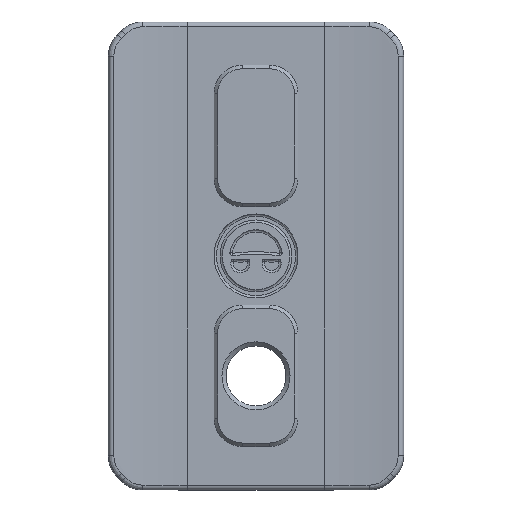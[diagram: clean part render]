
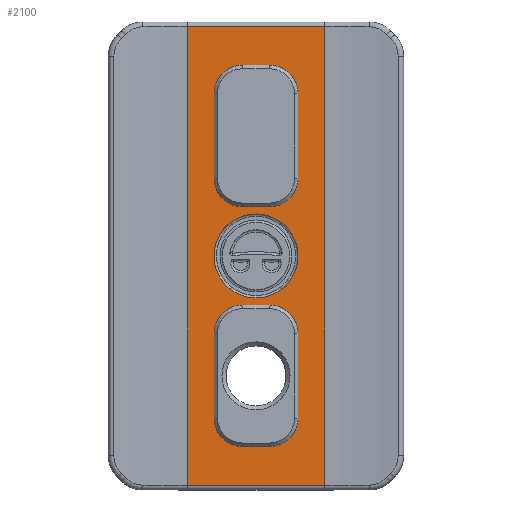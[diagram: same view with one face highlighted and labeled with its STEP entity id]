
A CAD part, top view. The second image highlights one B-rep face of the part: STEP entity #2100.
In plain terms, the highlighted planar face has unit normal (0, 0, 1).
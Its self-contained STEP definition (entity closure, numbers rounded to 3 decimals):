
#126=FACE_BOUND('',#397,.T.);
#127=FACE_BOUND('',#398,.T.);
#128=FACE_BOUND('',#399,.T.);
#199=PLANE('',#2283);
#251=FACE_OUTER_BOUND('',#396,.T.);
#396=EDGE_LOOP('',(#1549,#1550,#1551,#1552));
#397=EDGE_LOOP('',(#1553,#1554,#1555,#1556,#1557,#1558,#1559,#1560));
#398=EDGE_LOOP('',(#1561));
#399=EDGE_LOOP('',(#1562,#1563,#1564,#1565,#1566,#1567,#1568,#1569));
#525=CIRCLE('',#2244,2.38);
#526=CIRCLE('',#2247,2.38);
#535=CIRCLE('',#2266,2.38);
#536=CIRCLE('',#2269,2.38);
#538=CIRCLE('',#2274,2.38);
#539=CIRCLE('',#2277,2.38);
#540=CIRCLE('',#2279,2.38);
#541=CIRCLE('',#2282,2.38);
#542=CIRCLE('',#2284,3.5);
#677=LINE('',#3244,#797);
#681=LINE('',#3253,#801);
#702=LINE('',#3316,#822);
#705=LINE('',#3324,#825);
#709=LINE('',#3337,#829);
#712=LINE('',#3347,#832);
#714=LINE('',#3355,#834);
#715=LINE('',#3357,#835);
#716=LINE('',#3359,#836);
#717=LINE('',#3360,#837);
#718=LINE('',#3361,#838);
#719=LINE('',#3364,#839);
#797=VECTOR('',#2560,10.);
#801=VECTOR('',#2570,10.);
#822=VECTOR('',#2635,10.);
#825=VECTOR('',#2644,10.);
#829=VECTOR('',#2658,10.);
#832=VECTOR('',#2671,10.);
#834=VECTOR('',#2679,10.);
#835=VECTOR('',#2680,10.);
#836=VECTOR('',#2681,10.);
#837=VECTOR('',#2682,10.);
#838=VECTOR('',#2683,10.);
#839=VECTOR('',#2686,10.);
#916=VERTEX_POINT('',#3241);
#917=VERTEX_POINT('',#3243);
#918=VERTEX_POINT('',#3247);
#919=VERTEX_POINT('',#3251);
#920=VERTEX_POINT('',#3255);
#937=VERTEX_POINT('',#3308);
#938=VERTEX_POINT('',#3310);
#939=VERTEX_POINT('',#3314);
#940=VERTEX_POINT('',#3318);
#941=VERTEX_POINT('',#3322);
#943=VERTEX_POINT('',#3329);
#944=VERTEX_POINT('',#3331);
#945=VERTEX_POINT('',#3335);
#946=VERTEX_POINT('',#3341);
#947=VERTEX_POINT('',#3343);
#948=VERTEX_POINT('',#3349);
#949=VERTEX_POINT('',#3353);
#950=VERTEX_POINT('',#3354);
#951=VERTEX_POINT('',#3356);
#952=VERTEX_POINT('',#3358);
#953=VERTEX_POINT('',#3362);
#1114=EDGE_CURVE('',#916,#917,#677,.T.);
#1117=EDGE_CURVE('',#918,#916,#525,.F.);
#1119=EDGE_CURVE('',#919,#918,#681,.F.);
#1121=EDGE_CURVE('',#920,#919,#526,.F.);
#1147=EDGE_CURVE('',#937,#938,#535,.F.);
#1150=EDGE_CURVE('',#939,#937,#702,.T.);
#1152=EDGE_CURVE('',#940,#939,#536,.F.);
#1154=EDGE_CURVE('',#941,#940,#705,.T.);
#1157=EDGE_CURVE('',#943,#944,#538,.F.);
#1160=EDGE_CURVE('',#945,#943,#709,.F.);
#1161=EDGE_CURVE('',#917,#945,#539,.F.);
#1163=EDGE_CURVE('',#946,#947,#540,.F.);
#1165=EDGE_CURVE('',#938,#946,#712,.F.);
#1167=EDGE_CURVE('',#948,#941,#541,.F.);
#1168=EDGE_CURVE('',#949,#950,#714,.T.);
#1169=EDGE_CURVE('',#951,#950,#715,.T.);
#1170=EDGE_CURVE('',#952,#951,#716,.T.);
#1171=EDGE_CURVE('',#949,#952,#717,.T.);
#1172=EDGE_CURVE('',#947,#948,#718,.T.);
#1173=EDGE_CURVE('',#953,#953,#542,.T.);
#1174=EDGE_CURVE('',#944,#920,#719,.T.);
#1549=ORIENTED_EDGE('',*,*,#1168,.T.);
#1550=ORIENTED_EDGE('',*,*,#1169,.F.);
#1551=ORIENTED_EDGE('',*,*,#1170,.F.);
#1552=ORIENTED_EDGE('',*,*,#1171,.F.);
#1553=ORIENTED_EDGE('',*,*,#1165,.F.);
#1554=ORIENTED_EDGE('',*,*,#1147,.F.);
#1555=ORIENTED_EDGE('',*,*,#1150,.F.);
#1556=ORIENTED_EDGE('',*,*,#1152,.F.);
#1557=ORIENTED_EDGE('',*,*,#1154,.F.);
#1558=ORIENTED_EDGE('',*,*,#1167,.F.);
#1559=ORIENTED_EDGE('',*,*,#1172,.F.);
#1560=ORIENTED_EDGE('',*,*,#1163,.F.);
#1561=ORIENTED_EDGE('',*,*,#1173,.T.);
#1562=ORIENTED_EDGE('',*,*,#1160,.F.);
#1563=ORIENTED_EDGE('',*,*,#1161,.F.);
#1564=ORIENTED_EDGE('',*,*,#1114,.F.);
#1565=ORIENTED_EDGE('',*,*,#1117,.F.);
#1566=ORIENTED_EDGE('',*,*,#1119,.F.);
#1567=ORIENTED_EDGE('',*,*,#1121,.F.);
#1568=ORIENTED_EDGE('',*,*,#1174,.F.);
#1569=ORIENTED_EDGE('',*,*,#1157,.F.);
#2100=ADVANCED_FACE('',(#251,#126,#127,#128),#199,.T.);
#2244=AXIS2_PLACEMENT_3D('',#3249,#2565,#2566);
#2247=AXIS2_PLACEMENT_3D('',#3257,#2574,#2575);
#2266=AXIS2_PLACEMENT_3D('',#3311,#2629,#2630);
#2269=AXIS2_PLACEMENT_3D('',#3320,#2639,#2640);
#2274=AXIS2_PLACEMENT_3D('',#3332,#2652,#2653);
#2277=AXIS2_PLACEMENT_3D('',#3339,#2661,#2662);
#2279=AXIS2_PLACEMENT_3D('',#3344,#2666,#2667);
#2282=AXIS2_PLACEMENT_3D('',#3351,#2675,#2676);
#2283=AXIS2_PLACEMENT_3D('',#3352,#2677,#2678);
#2284=AXIS2_PLACEMENT_3D('',#3363,#2684,#2685);
#2560=DIRECTION('',(0.,-1.,0.));
#2565=DIRECTION('center_axis',(0.,0.,-1.));
#2566=DIRECTION('ref_axis',(-0.707,0.707,0.));
#2570=DIRECTION('',(1.,0.,0.));
#2574=DIRECTION('center_axis',(0.,0.,-1.));
#2575=DIRECTION('ref_axis',(0.707,0.707,0.));
#2629=DIRECTION('center_axis',(0.,0.,-1.));
#2630=DIRECTION('ref_axis',(-0.707,-0.707,0.));
#2635=DIRECTION('',(0.,-1.,0.));
#2639=DIRECTION('center_axis',(0.,0.,-1.));
#2640=DIRECTION('ref_axis',(-0.707,0.707,0.));
#2644=DIRECTION('',(-1.,0.,0.));
#2652=DIRECTION('center_axis',(0.,0.,-1.));
#2653=DIRECTION('ref_axis',(0.707,-0.707,0.));
#2658=DIRECTION('',(-1.,0.,0.));
#2661=DIRECTION('center_axis',(0.,0.,-1.));
#2662=DIRECTION('ref_axis',(-0.707,-0.707,0.));
#2666=DIRECTION('center_axis',(0.,0.,-1.));
#2667=DIRECTION('ref_axis',(0.707,-0.707,0.));
#2671=DIRECTION('',(-1.,0.,0.));
#2675=DIRECTION('center_axis',(0.,0.,-1.));
#2676=DIRECTION('ref_axis',(0.707,0.707,0.));
#2677=DIRECTION('center_axis',(0.,0.,1.));
#2678=DIRECTION('ref_axis',(1.,0.,0.));
#2679=DIRECTION('',(0.,-1.,0.));
#2680=DIRECTION('',(-1.,0.,0.));
#2681=DIRECTION('',(0.,-1.,0.));
#2682=DIRECTION('',(1.,0.,0.));
#2683=DIRECTION('',(0.,1.,0.));
#2684=DIRECTION('center_axis',(0.,0.,-1.));
#2685=DIRECTION('ref_axis',(-1.,0.,0.));
#2686=DIRECTION('',(0.,1.,0.));
#3241=CARTESIAN_POINT('',(-3.5,37.52,-2.8));
#3243=CARTESIAN_POINT('',(-3.5,30.48,-2.8));
#3244=CARTESIAN_POINT('',(-3.5,7.19,-2.8));
#3247=CARTESIAN_POINT('',(-1.12,39.9,-2.8));
#3249=CARTESIAN_POINT('Origin',(-1.12,37.52,-2.8));
#3251=CARTESIAN_POINT('',(1.12,39.9,-2.8));
#3253=CARTESIAN_POINT('',(-30.56,39.9,-2.8));
#3255=CARTESIAN_POINT('',(3.5,37.52,-2.8));
#3257=CARTESIAN_POINT('Origin',(1.12,37.52,-2.8));
#3308=CARTESIAN_POINT('',(-3.5,10.48,-2.8));
#3310=CARTESIAN_POINT('',(-1.12,8.1,-2.8));
#3311=CARTESIAN_POINT('Origin',(-1.12,10.48,-2.8));
#3314=CARTESIAN_POINT('',(-3.5,17.52,-2.8));
#3316=CARTESIAN_POINT('',(-3.5,-2.81,-2.8));
#3318=CARTESIAN_POINT('',(-1.12,19.9,-2.8));
#3320=CARTESIAN_POINT('Origin',(-1.12,17.52,-2.8));
#3322=CARTESIAN_POINT('',(1.12,19.9,-2.8));
#3324=CARTESIAN_POINT('',(-29.44,19.9,-2.8));
#3329=CARTESIAN_POINT('',(1.12,28.1,-2.8));
#3331=CARTESIAN_POINT('',(3.5,30.48,-2.8));
#3332=CARTESIAN_POINT('Origin',(1.12,30.48,-2.8));
#3335=CARTESIAN_POINT('',(-1.12,28.1,-2.8));
#3337=CARTESIAN_POINT('',(-29.44,28.1,-2.8));
#3339=CARTESIAN_POINT('Origin',(-1.12,30.48,-2.8));
#3341=CARTESIAN_POINT('',(1.12,8.1,-2.8));
#3343=CARTESIAN_POINT('',(3.5,10.48,-2.8));
#3344=CARTESIAN_POINT('Origin',(1.12,10.48,-2.8));
#3347=CARTESIAN_POINT('',(-29.44,8.1,-2.8));
#3349=CARTESIAN_POINT('',(3.5,17.52,-2.8));
#3351=CARTESIAN_POINT('Origin',(1.12,17.52,-2.8));
#3352=CARTESIAN_POINT('Origin',(-60.,-16.,-2.8));
#3353=CARTESIAN_POINT('',(-5.713,43.1,-2.8));
#3354=CARTESIAN_POINT('',(-5.713,4.9,-2.8));
#3355=CARTESIAN_POINT('',(-5.713,-76.,-2.8));
#3356=CARTESIAN_POINT('',(5.713,4.9,-2.8));
#3357=CARTESIAN_POINT('',(0.,4.9,-2.8));
#3358=CARTESIAN_POINT('',(5.713,43.1,-2.8));
#3359=CARTESIAN_POINT('',(5.713,-76.,-2.8));
#3360=CARTESIAN_POINT('',(0.,43.1,-2.8));
#3361=CARTESIAN_POINT('',(3.5,0.81,-2.8));
#3362=CARTESIAN_POINT('',(3.5,24.,-2.8));
#3363=CARTESIAN_POINT('Origin',(0.,24.,-2.8));
#3364=CARTESIAN_POINT('',(3.5,10.81,-2.8));
